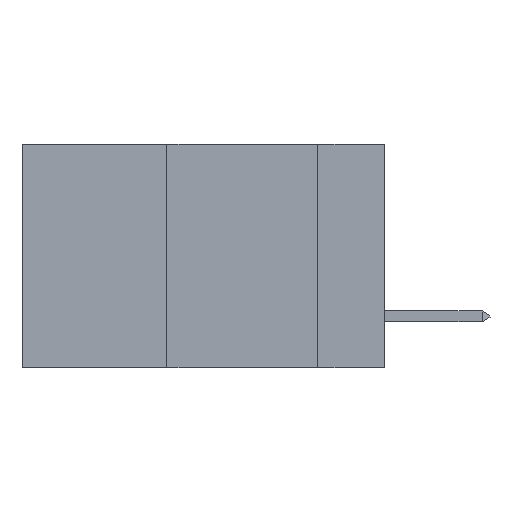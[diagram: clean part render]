
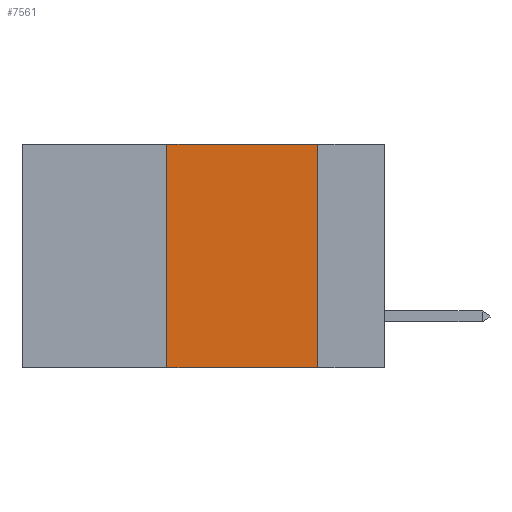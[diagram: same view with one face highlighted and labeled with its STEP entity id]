
A CAD part, left-side view. The second image highlights one B-rep face of the part: STEP entity #7561.
In plain terms, the highlighted planar face has unit normal (-1, 0, 0).
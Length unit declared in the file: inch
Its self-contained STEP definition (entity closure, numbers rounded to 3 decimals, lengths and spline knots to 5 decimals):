
#5 = EDGE_CURVE ( 'NONE', #8683, #8199, #6651, .T. ) ;
#192 = CARTESIAN_POINT ( 'NONE',  ( 0., 0.36, 0. ) ) ;
#343 = FACE_OUTER_BOUND ( 'NONE', #1672, .T. ) ;
#538 = CARTESIAN_POINT ( 'NONE',  ( 0., 0.11, 0. ) ) ;
#551 = DIRECTION ( 'NONE',  ( 0., -1., 0. ) ) ;
#781 = DIRECTION ( 'NONE',  ( 0., 0., -1. ) ) ;
#785 = CARTESIAN_POINT ( 'NONE',  ( 0., 0.6, 0. ) ) ;
#838 = CARTESIAN_POINT ( 'NONE',  ( 0., 0.6, 0. ) ) ;
#1066 = EDGE_CURVE ( 'NONE', #8683, #4278, #9647, .T. ) ;
#1656 = PLANE ( 'NONE',  #10438 ) ;
#1672 = EDGE_LOOP ( 'NONE', ( #3115, #5254, #2048, #8580 ) ) ;
#2048 = ORIENTED_EDGE ( 'NONE', *, *, #1066, .F. ) ;
#2368 = DIRECTION ( 'NONE',  ( 0., 0., -1. ) ) ;
#2369 = DIRECTION ( 'NONE',  ( 0., 0., 1. ) ) ;
#3012 = VECTOR ( 'NONE', #2369, 39.37008 ) ;
#3115 = ORIENTED_EDGE ( 'NONE', *, *, #7587, .F. ) ;
#3443 = EDGE_CURVE ( 'NONE', #4278, #6122, #9601, .T. ) ;
#3832 = DIRECTION ( 'NONE',  ( 1., 0., 0. ) ) ;
#4263 = VECTOR ( 'NONE', #4611, 39.37008 ) ;
#4278 = VERTEX_POINT ( 'NONE', #192 ) ;
#4549 = VECTOR ( 'NONE', #2368, 39.37008 ) ;
#4591 = CARTESIAN_POINT ( 'NONE',  ( 0., 0.36, 0. ) ) ;
#4611 = DIRECTION ( 'NONE',  ( 0., -1., 0. ) ) ;
#4641 = CARTESIAN_POINT ( 'NONE',  ( 0., 0.6, -0.37 ) ) ;
#4863 = CARTESIAN_POINT ( 'NONE',  ( 0., 0.36, -0.37 ) ) ;
#5133 = VECTOR ( 'NONE', #551, 39.37008 ) ;
#5254 = ORIENTED_EDGE ( 'NONE', *, *, #3443, .F. ) ;
#6122 = VERTEX_POINT ( 'NONE', #6749 ) ;
#6651 = LINE ( 'NONE', #4641, #4263 ) ;
#6749 = CARTESIAN_POINT ( 'NONE',  ( 0., 0.11, 0. ) ) ;
#6928 = LINE ( 'NONE', #538, #4549 ) ;
#7561 = ADVANCED_FACE ( 'NONE', ( #343 ), #1656, .F. ) ;
#7587 = EDGE_CURVE ( 'NONE', #6122, #8199, #6928, .T. ) ;
#8199 = VERTEX_POINT ( 'NONE', #8889 ) ;
#8580 = ORIENTED_EDGE ( 'NONE', *, *, #5, .T. ) ;
#8683 = VERTEX_POINT ( 'NONE', #4863 ) ;
#8889 = CARTESIAN_POINT ( 'NONE',  ( 0., 0.11, -0.37 ) ) ;
#9601 = LINE ( 'NONE', #838, #5133 ) ;
#9647 = LINE ( 'NONE', #4591, #3012 ) ;
#10438 = AXIS2_PLACEMENT_3D ( 'NONE', #785, #3832, #781 ) ;
